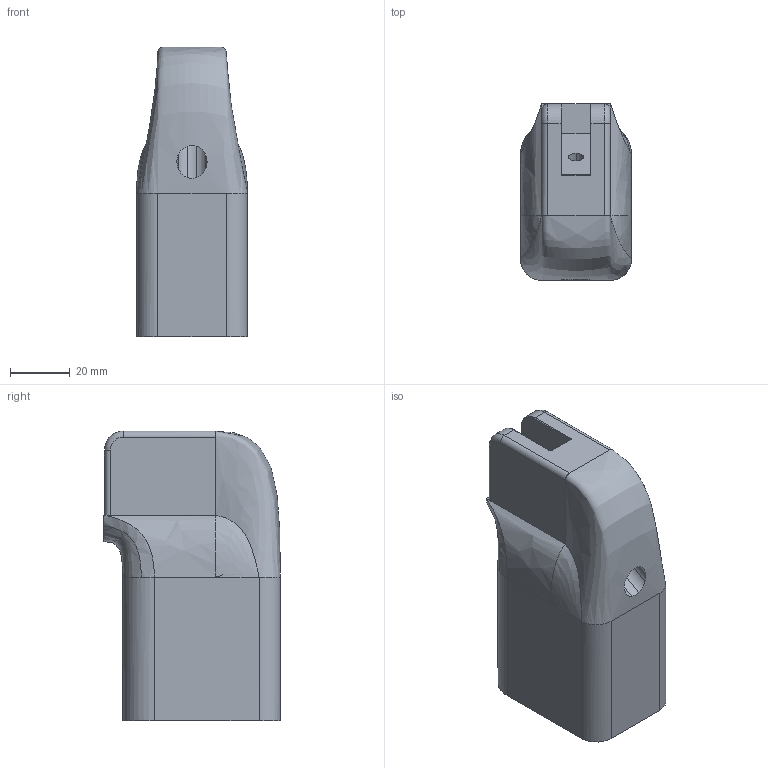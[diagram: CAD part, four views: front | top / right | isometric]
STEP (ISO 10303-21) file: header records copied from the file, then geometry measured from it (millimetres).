
FILE_DESCRIPTION (( 'STEP AP214' ), '1' );
FILE_NAME ('Sisyphus_Grip_Adapter.STEP', '2014-02-09T06:53:21', ( 'elpi' ), ( '' ), 'SwSTEP 2.0', 'SolidWorks 2013', '' );
FILE_SCHEMA (( 'AUTOMOTIVE_DESIGN' ));
Length unit declared in the file: millimetre
Products named in the file (1): Sisyphus_Grip_Adapter
Bounding box: 37.13 x 59.18 x 97.12 mm (x, y, z)
Volume: 113902 mm3; surface area: 31764.3 mm2
Topology: 1 solids, 1 shells, 149 faces, 407 edges, 261 vertices
Faces by surface type: cylinder 86, bspline 35, plane 22, torus 6
Entity records: 24205 total; most frequent: CARTESIAN_POINT 21084, ORIENTED_EDGE 810, DIRECTION 468, EDGE_CURVE 405, VERTEX_POINT 261, AXIS2_PLACEMENT_3D 164, EDGE_LOOP 154, ADVANCED_FACE 149
